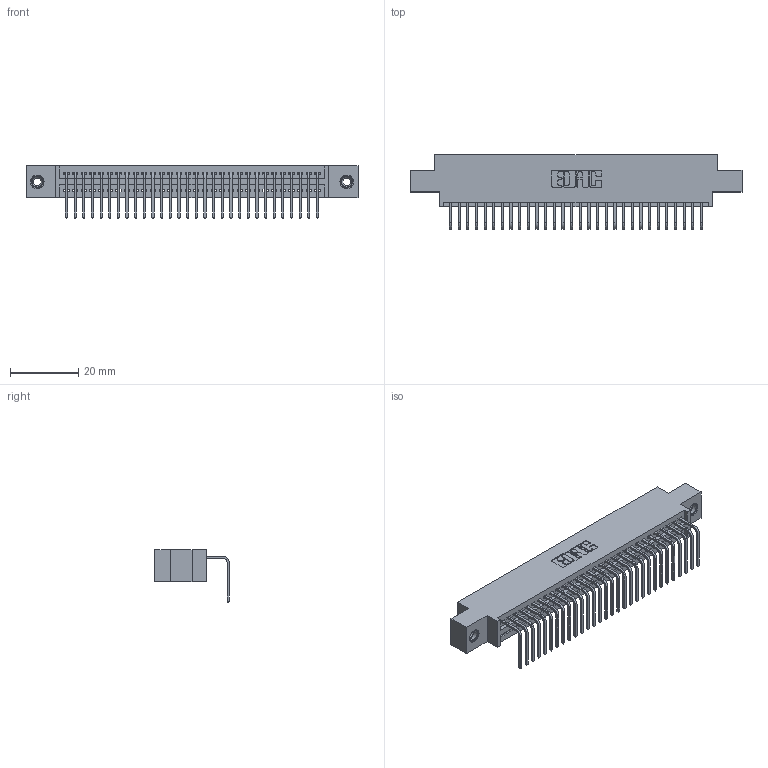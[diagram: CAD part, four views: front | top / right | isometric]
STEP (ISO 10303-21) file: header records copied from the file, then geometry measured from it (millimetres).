
FILE_DESCRIPTION (( 'STEP AP203' ), '1' );
FILE_NAME ('395-030-558-608.STEP', '2018-11-11T08:58:21', ( '' ), ( '' ), 'SwSTEP 2.0', 'SolidWorks 2016', '' );
FILE_SCHEMA (( 'CONFIG_CONTROL_DESIGN' ));
Length unit declared in the file: inch
Products named in the file (4): 345-292-001_558 Tail - 2; 395-030-558-608; 345-250-001_345-250-003-102; 345 Part_0.170 Offset - 0.156 Dia-TI
Assembly tree (33 placements, depth 2):
  395-030-558-608
    345 Part_0.170 Offset - 0.156 Dia-TI
    345-292-001_558 Tail - 2  x30
    345-250-001_345-250-003-102  x2
Bounding box: 97.41 x 21.83 x 15.37 mm (x, y, z)
Volume: 9133.8 mm3; surface area: 12707.9 mm2
Topology: 33 solids, 33 shells, 1990 faces, 5949 edges, 3918 vertices
Faces by surface type: plane 1376, cylinder 598, cone 12, torus 4
Entity records: 25596 total; most frequent: CARTESIAN_POINT 4417, ORIENTED_EDGE 4374, DIRECTION 3901, EDGE_CURVE 2187, LINE 1915, VECTOR 1915, VERTEX_POINT 1452, AXIS2_PLACEMENT_3D 993
